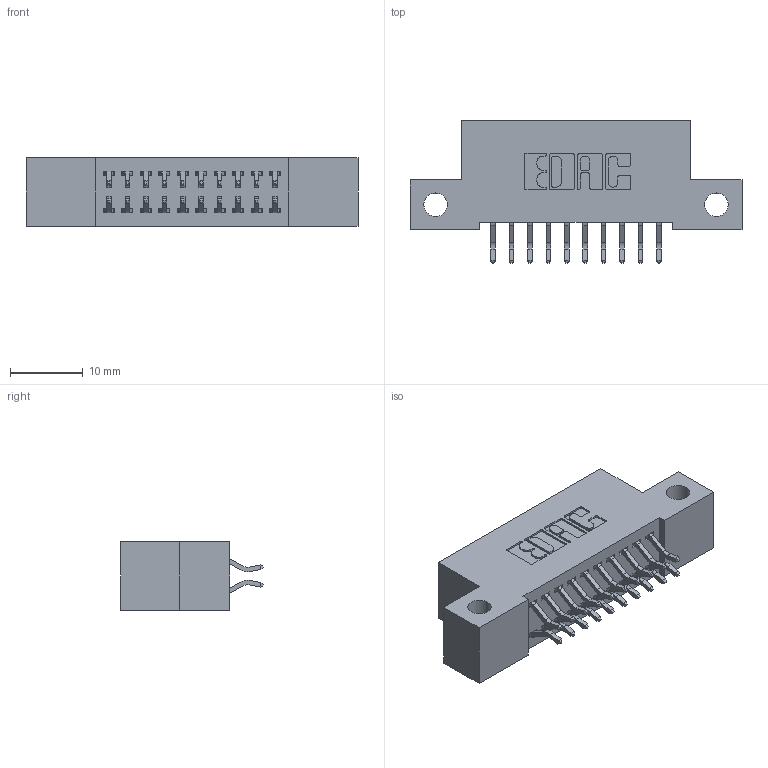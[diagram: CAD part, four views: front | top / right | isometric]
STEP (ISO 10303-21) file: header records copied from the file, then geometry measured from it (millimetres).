
FILE_DESCRIPTION (( 'STEP AP203' ), '1' );
FILE_NAME ('342-020-556-212.STEP', '2018-08-10T23:19:12', ( '' ), ( '' ), 'SwSTEP 2.0', 'SolidWorks 2016', '' );
FILE_SCHEMA (( 'CONFIG_CONTROL_DESIGN' ));
Length unit declared in the file: inch
Products named in the file (3): 345-292-001_556 Tail; 342-020-556-212; 342 Part_Side Mount
Assembly tree (21 placements, depth 2):
  342-020-556-212
    342 Part_Side Mount
    345-292-001_556 Tail  x20
Bounding box: 45.72 x 19.58 x 9.4 mm (x, y, z)
Volume: 3882 mm3; surface area: 5351.3 mm2
Topology: 21 solids, 21 shells, 1270 faces, 3759 edges, 2478 vertices
Faces by surface type: plane 866, cylinder 404
Entity records: 10663 total; most frequent: CARTESIAN_POINT 1818, ORIENTED_EDGE 1742, DIRECTION 1599, EDGE_CURVE 871, VECTOR 735, LINE 735, VERTEX_POINT 578, AXIS2_PLACEMENT_3D 432
